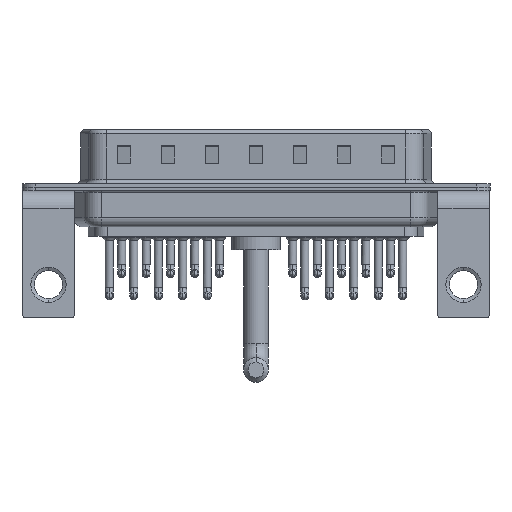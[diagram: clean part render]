
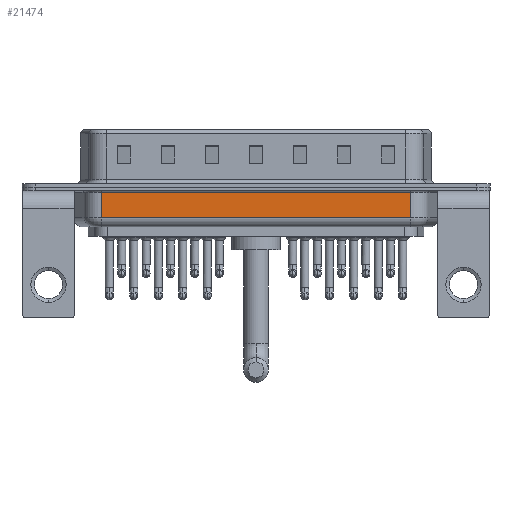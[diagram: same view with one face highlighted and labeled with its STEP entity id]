
A CAD part, front view. The second image highlights one B-rep face of the part: STEP entity #21474.
In plain terms, the highlighted planar face has unit normal (0, -1, 0).
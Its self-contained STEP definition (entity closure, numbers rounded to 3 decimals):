
#756 = VECTOR ( 'NONE', #3330, 1000. ) ;
#1179 = LINE ( 'NONE', #9431, #756 ) ;
#1730 = VECTOR ( 'NONE', #11357, 1000. ) ;
#2728 = CARTESIAN_POINT ( 'NONE',  ( 41.044, -5.35, -4.5 ) ) ;
#2858 = EDGE_CURVE ( 'NONE', #20252, #5316, #21327, .T. ) ;
#3330 = DIRECTION ( 'NONE',  ( 0., 0., 1. ) ) ;
#4899 = ORIENTED_EDGE ( 'NONE', *, *, #12725, .T. ) ;
#5316 = VERTEX_POINT ( 'NONE', #19029 ) ;
#5658 = FACE_OUTER_BOUND ( 'NONE', #11936, .T. ) ;
#6501 = VERTEX_POINT ( 'NONE', #26537 ) ;
#6865 = DIRECTION ( 'NONE',  ( 1., 0., 0. ) ) ;
#7822 = CARTESIAN_POINT ( 'NONE',  ( 6.006, -5.35, -4.5 ) ) ;
#9431 = CARTESIAN_POINT ( 'NONE',  ( 6.006, -5.35, -4.5 ) ) ;
#10018 = EDGE_CURVE ( 'NONE', #6501, #24624, #1179, .T. ) ;
#10489 = CARTESIAN_POINT ( 'NONE',  ( 6.006, -5.35, -0.65 ) ) ;
#11357 = DIRECTION ( 'NONE',  ( -1., 0., 0. ) ) ;
#11458 = AXIS2_PLACEMENT_3D ( 'NONE', #7822, #18132, #22077 ) ;
#11936 = EDGE_LOOP ( 'NONE', ( #21707, #4899, #21623, #23229 ) ) ;
#12725 = EDGE_CURVE ( 'NONE', #6501, #20252, #23299, .T. ) ;
#13536 = EDGE_CURVE ( 'NONE', #5316, #24624, #19384, .T. ) ;
#15101 = VECTOR ( 'NONE', #6865, 1000. ) ;
#15672 = PLANE ( 'NONE',  #11458 ) ;
#18132 = DIRECTION ( 'NONE',  ( 0., 1., 0. ) ) ;
#18755 = DIRECTION ( 'NONE',  ( 0., 0., 1. ) ) ;
#19029 = CARTESIAN_POINT ( 'NONE',  ( 41.044, -5.35, -0.65 ) ) ;
#19384 = LINE ( 'NONE', #23717, #1730 ) ;
#20252 = VERTEX_POINT ( 'NONE', #20719 ) ;
#20719 = CARTESIAN_POINT ( 'NONE',  ( 41.044, -5.35, -3.5 ) ) ;
#21327 = LINE ( 'NONE', #2728, #24259 ) ;
#21474 = ADVANCED_FACE ( 'NONE', ( #5658 ), #15672, .F. ) ;
#21623 = ORIENTED_EDGE ( 'NONE', *, *, #2858, .T. ) ;
#21707 = ORIENTED_EDGE ( 'NONE', *, *, #10018, .F. ) ;
#22077 = DIRECTION ( 'NONE',  ( 0., 0., 1. ) ) ;
#23229 = ORIENTED_EDGE ( 'NONE', *, *, #13536, .T. ) ;
#23299 = LINE ( 'NONE', #25463, #15101 ) ;
#23717 = CARTESIAN_POINT ( 'NONE',  ( 6.006, -5.35, -0.65 ) ) ;
#24259 = VECTOR ( 'NONE', #18755, 1000. ) ;
#24624 = VERTEX_POINT ( 'NONE', #10489 ) ;
#25463 = CARTESIAN_POINT ( 'NONE',  ( 6.006, -5.35, -3.5 ) ) ;
#26537 = CARTESIAN_POINT ( 'NONE',  ( 6.006, -5.35, -3.5 ) ) ;
